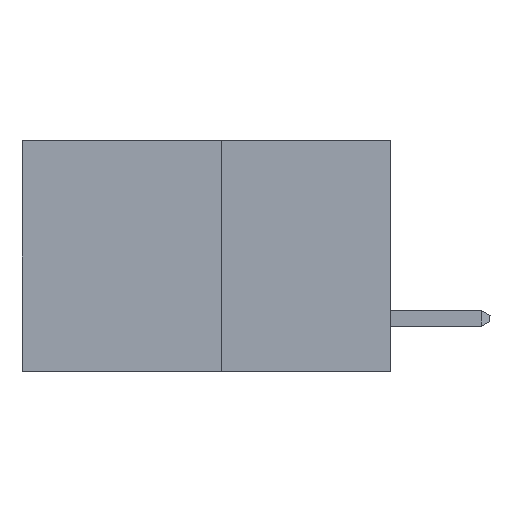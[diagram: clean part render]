
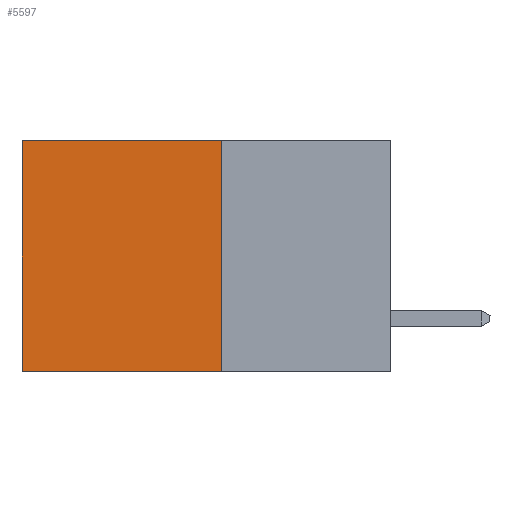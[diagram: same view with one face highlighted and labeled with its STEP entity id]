
A CAD part, left-side view. The second image highlights one B-rep face of the part: STEP entity #5597.
In plain terms, the highlighted planar face has unit normal (-1, 0, 0).
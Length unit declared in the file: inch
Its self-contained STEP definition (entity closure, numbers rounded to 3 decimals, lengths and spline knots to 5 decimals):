
#257 = VERTEX_POINT ( 'NONE', #4807 ) ;
#372 = CARTESIAN_POINT ( 'NONE',  ( 0.277, 0.59, 0. ) ) ;
#649 = CARTESIAN_POINT ( 'NONE',  ( 0.277, 0.27, 0. ) ) ;
#949 = CARTESIAN_POINT ( 'NONE',  ( 0.277, 0.27, -0.37 ) ) ;
#1019 = FACE_OUTER_BOUND ( 'NONE', #2024, .T. ) ;
#1067 = PLANE ( 'NONE',  #2325 ) ;
#1159 = CARTESIAN_POINT ( 'NONE',  ( 0.277, 0.27, -0.37 ) ) ;
#1398 = VECTOR ( 'NONE', #6990, 39.37008 ) ;
#1556 = DIRECTION ( 'NONE',  ( 0., 0., -1. ) ) ;
#1690 = CARTESIAN_POINT ( 'NONE',  ( 0.277, 0.59, -0.37 ) ) ;
#2024 = EDGE_LOOP ( 'NONE', ( #3459, #3487, #3495, #3503 ) ) ;
#2166 = DIRECTION ( 'NONE',  ( 1., 0., 0. ) ) ;
#2325 = AXIS2_PLACEMENT_3D ( 'NONE', #1159, #2166, #2859 ) ;
#2859 = DIRECTION ( 'NONE',  ( 0., 0., -1. ) ) ;
#3459 = ORIENTED_EDGE ( 'NONE', *, *, #5579, .T. ) ;
#3487 = ORIENTED_EDGE ( 'NONE', *, *, #7594, .F. ) ;
#3495 = ORIENTED_EDGE ( 'NONE', *, *, #6922, .F. ) ;
#3503 = ORIENTED_EDGE ( 'NONE', *, *, #7090, .T. ) ;
#3618 = VECTOR ( 'NONE', #5651, 39.37008 ) ;
#4029 = LINE ( 'NONE', #949, #3618 ) ;
#4050 = DIRECTION ( 'NONE',  ( 0., 1., 0. ) ) ;
#4398 = VERTEX_POINT ( 'NONE', #7278 ) ;
#4464 = CARTESIAN_POINT ( 'NONE',  ( 0.277, 0.27, -0.37 ) ) ;
#4587 = VERTEX_POINT ( 'NONE', #372 ) ;
#4643 = LINE ( 'NONE', #1690, #7636 ) ;
#4807 = CARTESIAN_POINT ( 'NONE',  ( 0.277, 0.59, -0.37 ) ) ;
#5579 = EDGE_CURVE ( 'NONE', #4587, #257, #4643, .T. ) ;
#5597 = ADVANCED_FACE ( 'NONE', ( #1019 ), #1067, .F. ) ;
#5651 = DIRECTION ( 'NONE',  ( 0., 1., 0. ) ) ;
#6172 = VECTOR ( 'NONE', #4050, 39.37008 ) ;
#6664 = LINE ( 'NONE', #4464, #1398 ) ;
#6687 = VERTEX_POINT ( 'NONE', #7737 ) ;
#6922 = EDGE_CURVE ( 'NONE', #6687, #4398, #6664, .T. ) ;
#6990 = DIRECTION ( 'NONE',  ( 0., 0., -1. ) ) ;
#7090 = EDGE_CURVE ( 'NONE', #6687, #4587, #7847, .T. ) ;
#7278 = CARTESIAN_POINT ( 'NONE',  ( 0.277, 0.27, -0.37 ) ) ;
#7594 = EDGE_CURVE ( 'NONE', #4398, #257, #4029, .T. ) ;
#7636 = VECTOR ( 'NONE', #1556, 39.37008 ) ;
#7737 = CARTESIAN_POINT ( 'NONE',  ( 0.277, 0.27, 0. ) ) ;
#7847 = LINE ( 'NONE', #649, #6172 ) ;
